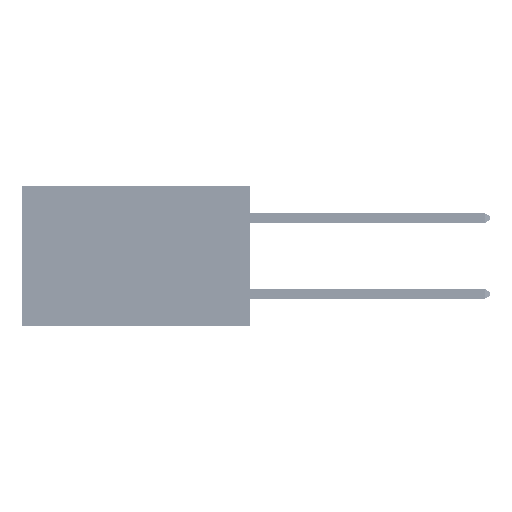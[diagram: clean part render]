
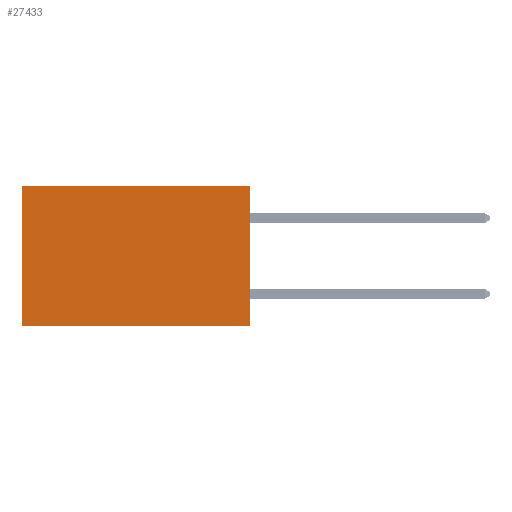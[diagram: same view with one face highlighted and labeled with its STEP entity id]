
A CAD part, left-side view. The second image highlights one B-rep face of the part: STEP entity #27433.
In plain terms, the highlighted planar face has unit normal (-1, 0, 0).
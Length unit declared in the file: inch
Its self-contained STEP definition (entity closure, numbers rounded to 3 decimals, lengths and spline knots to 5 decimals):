
#1741 = LINE ( 'NONE', #23964, #31526 ) ;
#2510 = LINE ( 'NONE', #15878, #17747 ) ;
#5187 = ORIENTED_EDGE ( 'NONE', *, *, #14679, .T. ) ;
#10044 = DIRECTION ( 'NONE',  ( 0., 0., -1. ) ) ;
#11070 = ORIENTED_EDGE ( 'NONE', *, *, #25151, .T. ) ;
#12832 = LINE ( 'NONE', #15886, #42508 ) ;
#13037 = CARTESIAN_POINT ( 'NONE',  ( 0.2875, 0.6, -0.37 ) ) ;
#14679 = EDGE_CURVE ( 'NONE', #25626, #40834, #12832, .T. ) ;
#15826 = AXIS2_PLACEMENT_3D ( 'NONE', #41729, #18505, #49850 ) ;
#15878 = CARTESIAN_POINT ( 'NONE',  ( 0.2875, 0., -0.37 ) ) ;
#15886 = CARTESIAN_POINT ( 'NONE',  ( 0.2875, 0.6, 0. ) ) ;
#16926 = EDGE_CURVE ( 'NONE', #35855, #45323, #45301, .T. ) ;
#17747 = VECTOR ( 'NONE', #42982, 39.37008 ) ;
#18505 = DIRECTION ( 'NONE',  ( 1., 0., 0. ) ) ;
#19049 = ORIENTED_EDGE ( 'NONE', *, *, #16926, .F. ) ;
#20229 = DIRECTION ( 'NONE',  ( 0., 1., 0. ) ) ;
#21565 = CARTESIAN_POINT ( 'NONE',  ( 0.2875, 0., 0. ) ) ;
#23964 = CARTESIAN_POINT ( 'NONE',  ( 0.2875, 0., 0. ) ) ;
#25151 = EDGE_CURVE ( 'NONE', #35855, #25626, #1741, .T. ) ;
#25626 = VERTEX_POINT ( 'NONE', #35040 ) ;
#27002 = PLANE ( 'NONE',  #15826 ) ;
#27433 = ADVANCED_FACE ( 'NONE', ( #37337 ), #27002, .F. ) ;
#27768 = DIRECTION ( 'NONE',  ( 0., 0., -1. ) ) ;
#29573 = EDGE_CURVE ( 'NONE', #45323, #40834, #2510, .T. ) ;
#31235 = CARTESIAN_POINT ( 'NONE',  ( 0.2875, 0., 0. ) ) ;
#31526 = VECTOR ( 'NONE', #20229, 39.37008 ) ;
#35040 = CARTESIAN_POINT ( 'NONE',  ( 0.2875, 0.6, 0. ) ) ;
#35855 = VERTEX_POINT ( 'NONE', #31235 ) ;
#37337 = FACE_OUTER_BOUND ( 'NONE', #45345, .T. ) ;
#40834 = VERTEX_POINT ( 'NONE', #13037 ) ;
#41729 = CARTESIAN_POINT ( 'NONE',  ( 0.2875, 0., 0. ) ) ;
#42508 = VECTOR ( 'NONE', #27768, 39.37008 ) ;
#42982 = DIRECTION ( 'NONE',  ( 0., 1., 0. ) ) ;
#44715 = VECTOR ( 'NONE', #10044, 39.37008 ) ;
#45301 = LINE ( 'NONE', #21565, #44715 ) ;
#45323 = VERTEX_POINT ( 'NONE', #46683 ) ;
#45345 = EDGE_LOOP ( 'NONE', ( #5187, #49380, #19049, #11070 ) ) ;
#46683 = CARTESIAN_POINT ( 'NONE',  ( 0.2875, 0., -0.37 ) ) ;
#49380 = ORIENTED_EDGE ( 'NONE', *, *, #29573, .F. ) ;
#49850 = DIRECTION ( 'NONE',  ( 0., 0., -1. ) ) ;
